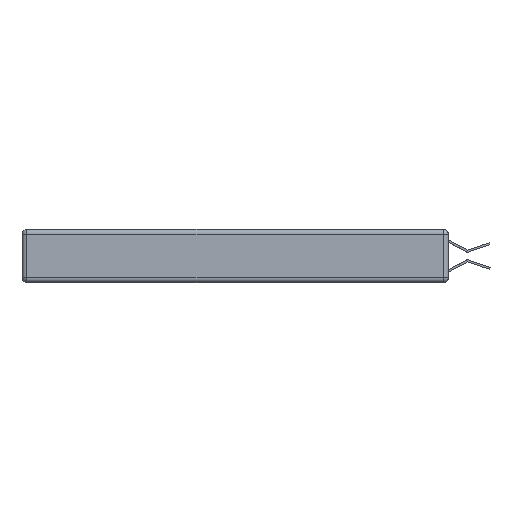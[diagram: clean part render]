
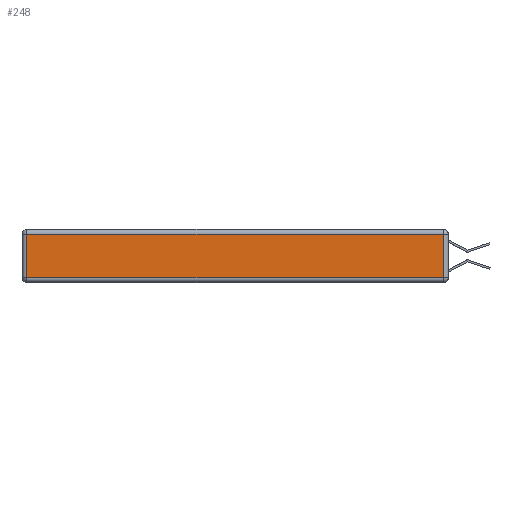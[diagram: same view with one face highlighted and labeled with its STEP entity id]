
A CAD part, left-side view. The second image highlights one B-rep face of the part: STEP entity #248.
In plain terms, the highlighted planar face has unit normal (-1, 0, 0).
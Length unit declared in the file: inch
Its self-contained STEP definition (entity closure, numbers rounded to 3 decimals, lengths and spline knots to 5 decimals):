
#248 = ADVANCED_FACE ( 'NONE', ( #3249 ), #8591, .T. ) ;
#1932 = DIRECTION ( 'NONE',  ( -1., 0., 0. ) ) ;
#1988 = DIRECTION ( 'NONE',  ( 0., 0., -1. ) ) ;
#1989 = DIRECTION ( 'NONE',  ( 0., 0., 1. ) ) ;
#2410 = ORIENTED_EDGE ( 'NONE', *, *, #7088, .T. ) ;
#2975 = VERTEX_POINT ( 'NONE', #3025 ) ;
#3025 = CARTESIAN_POINT ( 'NONE',  ( 0., 2.72, -0.03 ) ) ;
#3249 = FACE_OUTER_BOUND ( 'NONE', #15727, .T. ) ;
#3339 = CARTESIAN_POINT ( 'NONE',  ( 0., 0.03, -0.343 ) ) ;
#3578 = VERTEX_POINT ( 'NONE', #6915 ) ;
#4079 = DIRECTION ( 'NONE',  ( 0., 1., 0. ) ) ;
#5064 = VECTOR ( 'NONE', #1988, 39.37008 ) ;
#5285 = EDGE_CURVE ( 'NONE', #15490, #12065, #15547, .T. ) ;
#5595 = CARTESIAN_POINT ( 'NONE',  ( 0., 0.03, -0.313 ) ) ;
#6021 = VECTOR ( 'NONE', #4079, 39.37008 ) ;
#6915 = CARTESIAN_POINT ( 'NONE',  ( 0., 0.03, -0.03 ) ) ;
#7088 = EDGE_CURVE ( 'NONE', #3578, #2975, #10895, .T. ) ;
#7437 = CARTESIAN_POINT ( 'NONE',  ( 0., 0., -0.343 ) ) ;
#7846 = ORIENTED_EDGE ( 'NONE', *, *, #5285, .T. ) ;
#8001 = ORIENTED_EDGE ( 'NONE', *, *, #9939, .T. ) ;
#8056 = DIRECTION ( 'NONE',  ( 0., -1., 0. ) ) ;
#8365 = VECTOR ( 'NONE', #10175, 39.37008 ) ;
#8572 = LINE ( 'NONE', #3339, #8365 ) ;
#8591 = PLANE ( 'NONE',  #15545 ) ;
#9939 = EDGE_CURVE ( 'NONE', #2975, #15490, #14251, .T. ) ;
#9968 = ORIENTED_EDGE ( 'NONE', *, *, #17633, .T. ) ;
#10175 = DIRECTION ( 'NONE',  ( 0., 0., 1. ) ) ;
#10206 = CARTESIAN_POINT ( 'NONE',  ( 0., 2.72, -0.343 ) ) ;
#10895 = LINE ( 'NONE', #12424, #6021 ) ;
#11876 = VECTOR ( 'NONE', #8056, 39.37008 ) ;
#12065 = VERTEX_POINT ( 'NONE', #5595 ) ;
#12424 = CARTESIAN_POINT ( 'NONE',  ( 0., 2.75, -0.03 ) ) ;
#14251 = LINE ( 'NONE', #10206, #5064 ) ;
#15490 = VERTEX_POINT ( 'NONE', #16807 ) ;
#15545 = AXIS2_PLACEMENT_3D ( 'NONE', #7437, #1932, #1989 ) ;
#15547 = LINE ( 'NONE', #16271, #11876 ) ;
#15727 = EDGE_LOOP ( 'NONE', ( #7846, #9968, #2410, #8001 ) ) ;
#16271 = CARTESIAN_POINT ( 'NONE',  ( 0., 0., -0.313 ) ) ;
#16807 = CARTESIAN_POINT ( 'NONE',  ( 0., 2.72, -0.313 ) ) ;
#17633 = EDGE_CURVE ( 'NONE', #12065, #3578, #8572, .T. ) ;
